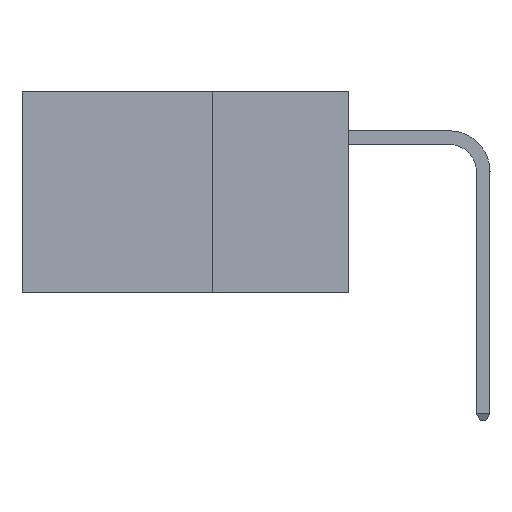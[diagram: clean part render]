
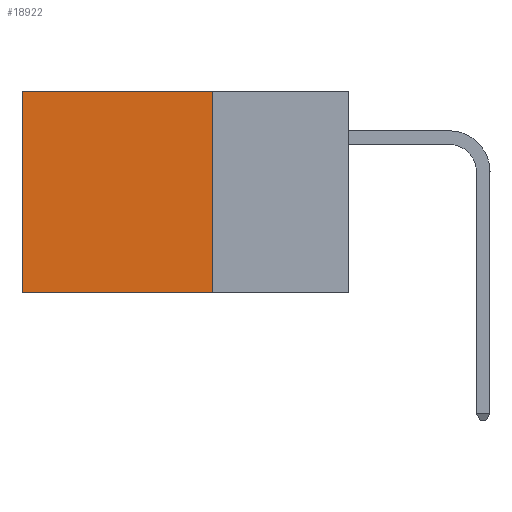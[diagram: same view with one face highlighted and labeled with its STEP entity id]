
A CAD part, left-side view. The second image highlights one B-rep face of the part: STEP entity #18922.
In plain terms, the highlighted planar face has unit normal (-1, 0, 0).
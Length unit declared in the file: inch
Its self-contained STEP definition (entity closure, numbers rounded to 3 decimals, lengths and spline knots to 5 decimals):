
#2134 = VERTEX_POINT ( 'NONE', #29296 ) ;
#2270 = VERTEX_POINT ( 'NONE', #30336 ) ;
#5376 = DIRECTION ( 'NONE',  ( 0., 1., 0. ) ) ;
#5711 = CARTESIAN_POINT ( 'NONE',  ( 0.2875, 0.6, 0. ) ) ;
#6021 = EDGE_LOOP ( 'NONE', ( #11166, #31111, #26622, #11029 ) ) ;
#6053 = VECTOR ( 'NONE', #23936, 39.37008 ) ;
#8192 = DIRECTION ( 'NONE',  ( 0., 1., 0. ) ) ;
#8304 = CARTESIAN_POINT ( 'NONE',  ( 0.2875, 0.6, -0.37 ) ) ;
#8725 = EDGE_CURVE ( 'NONE', #2134, #2270, #16482, .T. ) ;
#10297 = CARTESIAN_POINT ( 'NONE',  ( 0.2875, 0.25, 0. ) ) ;
#11029 = ORIENTED_EDGE ( 'NONE', *, *, #29358, .T. ) ;
#11166 = ORIENTED_EDGE ( 'NONE', *, *, #11732, .T. ) ;
#11732 = EDGE_CURVE ( 'NONE', #11959, #25373, #32702, .T. ) ;
#11959 = VERTEX_POINT ( 'NONE', #29832 ) ;
#12697 = CARTESIAN_POINT ( 'NONE',  ( 0.2875, 0.25, 0. ) ) ;
#12973 = DIRECTION ( 'NONE',  ( 1., 0., 0. ) ) ;
#14272 = VECTOR ( 'NONE', #5376, 39.37008 ) ;
#15953 = CARTESIAN_POINT ( 'NONE',  ( 0.2875, 0.25, 0. ) ) ;
#16482 = LINE ( 'NONE', #12697, #27773 ) ;
#18922 = ADVANCED_FACE ( 'NONE', ( #28972 ), #23211, .F. ) ;
#21051 = CARTESIAN_POINT ( 'NONE',  ( 0.2875, 0.25, -0.37 ) ) ;
#21716 = VECTOR ( 'NONE', #8192, 39.37008 ) ;
#22515 = LINE ( 'NONE', #15953, #21716 ) ;
#23211 = PLANE ( 'NONE',  #30531 ) ;
#23936 = DIRECTION ( 'NONE',  ( 0., 0., -1. ) ) ;
#25303 = EDGE_CURVE ( 'NONE', #2270, #25373, #27168, .T. ) ;
#25373 = VERTEX_POINT ( 'NONE', #8304 ) ;
#26622 = ORIENTED_EDGE ( 'NONE', *, *, #8725, .F. ) ;
#27168 = LINE ( 'NONE', #21051, #14272 ) ;
#27773 = VECTOR ( 'NONE', #28211, 39.37008 ) ;
#28211 = DIRECTION ( 'NONE',  ( 0., 0., -1. ) ) ;
#28972 = FACE_OUTER_BOUND ( 'NONE', #6021, .T. ) ;
#29296 = CARTESIAN_POINT ( 'NONE',  ( 0.2875, 0.25, 0. ) ) ;
#29358 = EDGE_CURVE ( 'NONE', #2134, #11959, #22515, .T. ) ;
#29832 = CARTESIAN_POINT ( 'NONE',  ( 0.2875, 0.6, 0. ) ) ;
#30336 = CARTESIAN_POINT ( 'NONE',  ( 0.2875, 0.25, -0.37 ) ) ;
#30531 = AXIS2_PLACEMENT_3D ( 'NONE', #10297, #12973, #30884 ) ;
#30884 = DIRECTION ( 'NONE',  ( 0., 0., -1. ) ) ;
#31111 = ORIENTED_EDGE ( 'NONE', *, *, #25303, .F. ) ;
#32702 = LINE ( 'NONE', #5711, #6053 ) ;
